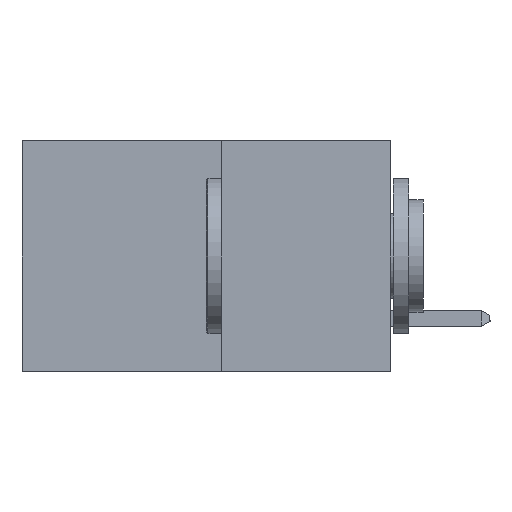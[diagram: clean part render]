
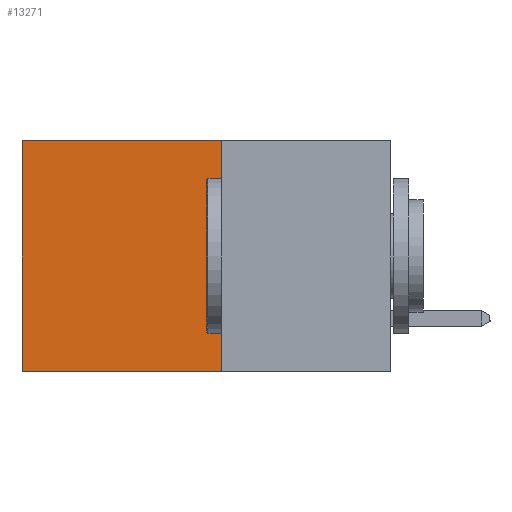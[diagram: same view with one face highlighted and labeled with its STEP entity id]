
A CAD part, left-side view. The second image highlights one B-rep face of the part: STEP entity #13271.
In plain terms, the highlighted planar face has unit normal (-1, 0, 0).
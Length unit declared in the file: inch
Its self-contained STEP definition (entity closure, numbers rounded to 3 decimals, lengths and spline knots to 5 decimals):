
#1097 = EDGE_CURVE ( 'NONE', #12652, #8138, #11310, .T. ) ;
#2217 = ORIENTED_EDGE ( 'NONE', *, *, #1097, .T. ) ;
#3156 = PLANE ( 'NONE',  #13596 ) ;
#3588 = CARTESIAN_POINT ( 'NONE',  ( 0.277, 0.27, -0.37 ) ) ;
#3593 = EDGE_CURVE ( 'NONE', #8138, #9700, #11580, .T. ) ;
#4042 = EDGE_LOOP ( 'NONE', ( #10912, #10188, #6533, #2217 ) ) ;
#4198 = EDGE_CURVE ( 'NONE', #5467, #9700, #13397, .T. ) ;
#4300 = DIRECTION ( 'NONE',  ( 0., 0., -1. ) ) ;
#4471 = VECTOR ( 'NONE', #6070, 39.37008 ) ;
#5247 = VECTOR ( 'NONE', #12825, 39.37008 ) ;
#5467 = VERTEX_POINT ( 'NONE', #11883 ) ;
#5724 = FACE_OUTER_BOUND ( 'NONE', #4042, .T. ) ;
#5791 = CARTESIAN_POINT ( 'NONE',  ( 0.277, 0.59, -0.37 ) ) ;
#6070 = DIRECTION ( 'NONE',  ( 0., 1., 0. ) ) ;
#6296 = CARTESIAN_POINT ( 'NONE',  ( 0.277, 0.27, 0. ) ) ;
#6533 = ORIENTED_EDGE ( 'NONE', *, *, #7015, .F. ) ;
#7015 = EDGE_CURVE ( 'NONE', #12652, #5467, #13786, .T. ) ;
#7840 = DIRECTION ( 'NONE',  ( 0., 0., -1. ) ) ;
#7882 = CARTESIAN_POINT ( 'NONE',  ( 0.277, 0.59, -0.37 ) ) ;
#8001 = DIRECTION ( 'NONE',  ( 0., 1., 0. ) ) ;
#8138 = VERTEX_POINT ( 'NONE', #8467 ) ;
#8467 = CARTESIAN_POINT ( 'NONE',  ( 0.277, 0.59, 0. ) ) ;
#8752 = VECTOR ( 'NONE', #7840, 39.37008 ) ;
#8800 = VECTOR ( 'NONE', #8001, 39.37008 ) ;
#9700 = VERTEX_POINT ( 'NONE', #5791 ) ;
#10188 = ORIENTED_EDGE ( 'NONE', *, *, #4198, .F. ) ;
#10786 = DIRECTION ( 'NONE',  ( 1., 0., 0. ) ) ;
#10912 = ORIENTED_EDGE ( 'NONE', *, *, #3593, .T. ) ;
#11310 = LINE ( 'NONE', #12806, #8800 ) ;
#11580 = LINE ( 'NONE', #7882, #8752 ) ;
#11883 = CARTESIAN_POINT ( 'NONE',  ( 0.277, 0.27, -0.37 ) ) ;
#12652 = VERTEX_POINT ( 'NONE', #6296 ) ;
#12806 = CARTESIAN_POINT ( 'NONE',  ( 0.277, 0.27, 0. ) ) ;
#12825 = DIRECTION ( 'NONE',  ( 0., 0., -1. ) ) ;
#13271 = ADVANCED_FACE ( 'NONE', ( #5724 ), #3156, .F. ) ;
#13397 = LINE ( 'NONE', #3588, #4471 ) ;
#13596 = AXIS2_PLACEMENT_3D ( 'NONE', #13957, #10786, #4300 ) ;
#13786 = LINE ( 'NONE', #14160, #5247 ) ;
#13957 = CARTESIAN_POINT ( 'NONE',  ( 0.277, 0.27, -0.37 ) ) ;
#14160 = CARTESIAN_POINT ( 'NONE',  ( 0.277, 0.27, -0.37 ) ) ;
